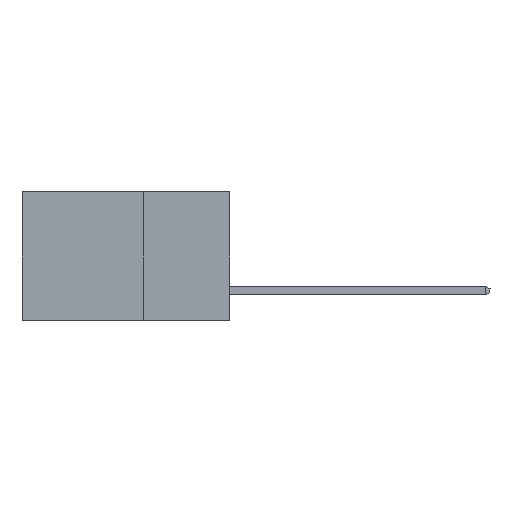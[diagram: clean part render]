
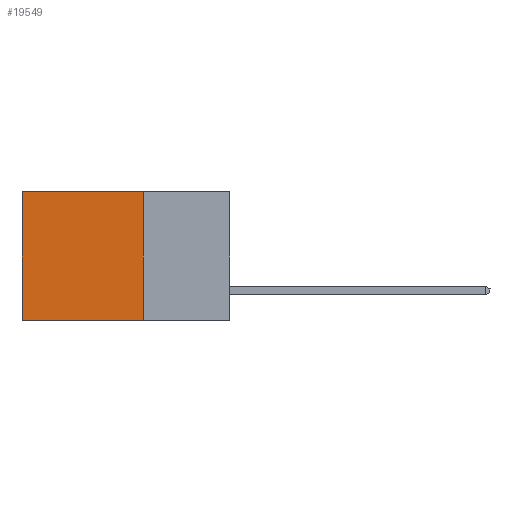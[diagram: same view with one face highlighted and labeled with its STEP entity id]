
A CAD part, left-side view. The second image highlights one B-rep face of the part: STEP entity #19549.
In plain terms, the highlighted planar face has unit normal (-1, 0, 0).
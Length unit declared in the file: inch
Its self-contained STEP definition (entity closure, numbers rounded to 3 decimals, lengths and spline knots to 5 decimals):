
#1806 = EDGE_CURVE ( 'NONE', #19276, #16887, #6850, .T. ) ;
#3031 = CARTESIAN_POINT ( 'NONE',  ( 0.2615, 0.25, -0.37 ) ) ;
#3522 = VERTEX_POINT ( 'NONE', #8368 ) ;
#3769 = CARTESIAN_POINT ( 'NONE',  ( 0.2615, 0.25, -0.37 ) ) ;
#3886 = ORIENTED_EDGE ( 'NONE', *, *, #18694, .F. ) ;
#4229 = LINE ( 'NONE', #10214, #11865 ) ;
#4922 = FACE_OUTER_BOUND ( 'NONE', #12969, .T. ) ;
#5209 = CARTESIAN_POINT ( 'NONE',  ( 0.2615, 0.25, 0. ) ) ;
#6075 = ORIENTED_EDGE ( 'NONE', *, *, #19845, .T. ) ;
#6133 = CARTESIAN_POINT ( 'NONE',  ( 0.2615, 0.25, 0. ) ) ;
#6329 = PLANE ( 'NONE',  #7734 ) ;
#6850 = LINE ( 'NONE', #3031, #16647 ) ;
#7086 = CARTESIAN_POINT ( 'NONE',  ( 0.2615, 0.6, 0. ) ) ;
#7734 = AXIS2_PLACEMENT_3D ( 'NONE', #9518, #10842, #12473 ) ;
#8368 = CARTESIAN_POINT ( 'NONE',  ( 0.2615, 0.6, -0.37 ) ) ;
#8513 = LINE ( 'NONE', #5209, #11720 ) ;
#9518 = CARTESIAN_POINT ( 'NONE',  ( 0.2615, 0.25, -0.37 ) ) ;
#10214 = CARTESIAN_POINT ( 'NONE',  ( 0.2615, 0.6, -0.37 ) ) ;
#10317 = DIRECTION ( 'NONE',  ( 0., 0., -1. ) ) ;
#10842 = DIRECTION ( 'NONE',  ( 1., 0., 0. ) ) ;
#10878 = EDGE_CURVE ( 'NONE', #19276, #13580, #8513, .T. ) ;
#11720 = VECTOR ( 'NONE', #13236, 39.37008 ) ;
#11865 = VECTOR ( 'NONE', #10317, 39.37008 ) ;
#12473 = DIRECTION ( 'NONE',  ( 0., 0., -1. ) ) ;
#12969 = EDGE_LOOP ( 'NONE', ( #6075, #3886, #17783, #14730 ) ) ;
#13236 = DIRECTION ( 'NONE',  ( 0., 1., 0. ) ) ;
#13580 = VERTEX_POINT ( 'NONE', #7086 ) ;
#14730 = ORIENTED_EDGE ( 'NONE', *, *, #10878, .T. ) ;
#15773 = VECTOR ( 'NONE', #19118, 39.37008 ) ;
#16072 = LINE ( 'NONE', #17382, #15773 ) ;
#16647 = VECTOR ( 'NONE', #18048, 39.37008 ) ;
#16887 = VERTEX_POINT ( 'NONE', #3769 ) ;
#17382 = CARTESIAN_POINT ( 'NONE',  ( 0.2615, 0.25, -0.37 ) ) ;
#17783 = ORIENTED_EDGE ( 'NONE', *, *, #1806, .F. ) ;
#18048 = DIRECTION ( 'NONE',  ( 0., 0., -1. ) ) ;
#18694 = EDGE_CURVE ( 'NONE', #16887, #3522, #16072, .T. ) ;
#19118 = DIRECTION ( 'NONE',  ( 0., 1., 0. ) ) ;
#19276 = VERTEX_POINT ( 'NONE', #6133 ) ;
#19549 = ADVANCED_FACE ( 'NONE', ( #4922 ), #6329, .F. ) ;
#19845 = EDGE_CURVE ( 'NONE', #13580, #3522, #4229, .T. ) ;
